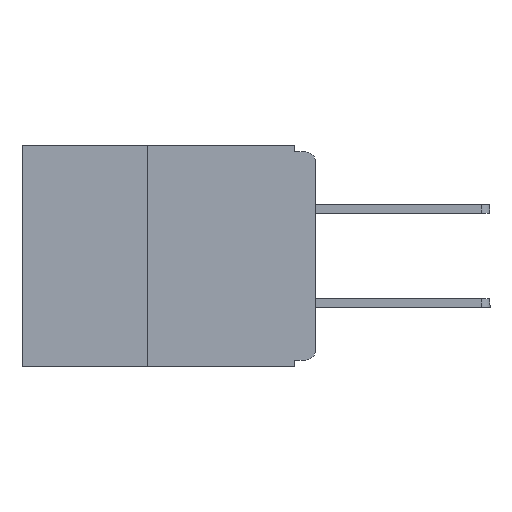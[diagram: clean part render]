
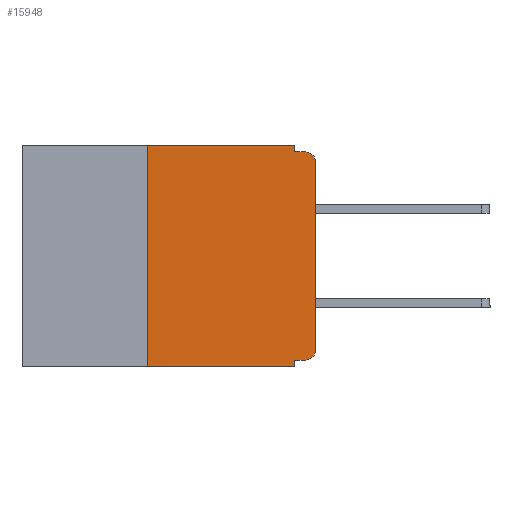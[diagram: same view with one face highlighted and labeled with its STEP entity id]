
A CAD part, left-side view. The second image highlights one B-rep face of the part: STEP entity #15948.
In plain terms, the highlighted planar face has unit normal (-1, 0, 0).
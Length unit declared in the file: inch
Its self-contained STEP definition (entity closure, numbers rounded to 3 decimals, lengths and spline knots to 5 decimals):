
#12 = ORIENTED_EDGE ( 'NONE', *, *, #6398, .T. ) ;
#51 = AXIS2_PLACEMENT_3D ( 'NONE', #2650, #11735, #3995 ) ;
#487 = LINE ( 'NONE', #12885, #13977 ) ;
#543 = CARTESIAN_POINT ( 'NONE',  ( 0., 0.031, -0.32 ) ) ;
#725 = EDGE_CURVE ( 'NONE', #6423, #3817, #10867, .T. ) ;
#857 = CARTESIAN_POINT ( 'NONE',  ( 0., 0.031, -0.33 ) ) ;
#880 = CARTESIAN_POINT ( 'NONE',  ( 0., 0., -0.01 ) ) ;
#1015 = VERTEX_POINT ( 'NONE', #11049 ) ;
#1126 = EDGE_CURVE ( 'NONE', #16452, #16335, #16360, .T. ) ;
#1258 = VERTEX_POINT ( 'NONE', #5091 ) ;
#1505 = VECTOR ( 'NONE', #9692, 39.37008 ) ;
#2023 = VERTEX_POINT ( 'NONE', #8123 ) ;
#2513 = DIRECTION ( 'NONE',  ( 0., 0., 1. ) ) ;
#2650 = CARTESIAN_POINT ( 'NONE',  ( 0., 0.015, -0.025 ) ) ;
#2837 = ORIENTED_EDGE ( 'NONE', *, *, #14425, .T. ) ;
#2912 = CARTESIAN_POINT ( 'NONE',  ( 0., 0.437, -0.33 ) ) ;
#3215 = DIRECTION ( 'NONE',  ( 0., 0., -1. ) ) ;
#3706 = EDGE_CURVE ( 'NONE', #16335, #1015, #5524, .T. ) ;
#3817 = VERTEX_POINT ( 'NONE', #857 ) ;
#3995 = DIRECTION ( 'NONE',  ( 0., 0., -1. ) ) ;
#4114 = CARTESIAN_POINT ( 'NONE',  ( 0., 0., 0. ) ) ;
#4115 = VERTEX_POINT ( 'NONE', #8576 ) ;
#4222 = VECTOR ( 'NONE', #12394, 39.37008 ) ;
#4335 = ORIENTED_EDGE ( 'NONE', *, *, #16655, .T. ) ;
#4448 = ORIENTED_EDGE ( 'NONE', *, *, #15796, .F. ) ;
#4653 = FACE_OUTER_BOUND ( 'NONE', #13528, .T. ) ;
#4668 = EDGE_CURVE ( 'NONE', #1015, #14729, #10681, .T. ) ;
#4706 = DIRECTION ( 'NONE',  ( 0., 0., 1. ) ) ;
#4980 = VECTOR ( 'NONE', #2513, 39.37008 ) ;
#5091 = CARTESIAN_POINT ( 'NONE',  ( 0., 0., -0.025 ) ) ;
#5524 = LINE ( 'NONE', #9822, #1505 ) ;
#6228 = DIRECTION ( 'NONE',  ( -1., 0., 0. ) ) ;
#6257 = CARTESIAN_POINT ( 'NONE',  ( 0., 0.437, 0. ) ) ;
#6385 = CARTESIAN_POINT ( 'NONE',  ( 0., 0.437, 0. ) ) ;
#6398 = EDGE_CURVE ( 'NONE', #4115, #1258, #11850, .T. ) ;
#6423 = VERTEX_POINT ( 'NONE', #543 ) ;
#6607 = ORIENTED_EDGE ( 'NONE', *, *, #10593, .F. ) ;
#6704 = DIRECTION ( 'NONE',  ( 0., -1., 0. ) ) ;
#7155 = CARTESIAN_POINT ( 'NONE',  ( 0., 0.031, 0. ) ) ;
#7385 = CARTESIAN_POINT ( 'NONE',  ( 0., 0.25, 0. ) ) ;
#7498 = VECTOR ( 'NONE', #11972, 39.37008 ) ;
#7620 = DIRECTION ( 'NONE',  ( 0., 0., -1. ) ) ;
#8123 = CARTESIAN_POINT ( 'NONE',  ( 0., 0.25, -0.33 ) ) ;
#8529 = ORIENTED_EDGE ( 'NONE', *, *, #15371, .T. ) ;
#8576 = CARTESIAN_POINT ( 'NONE',  ( 0., 0., -0.305 ) ) ;
#8855 = ORIENTED_EDGE ( 'NONE', *, *, #725, .F. ) ;
#9044 = DIRECTION ( 'NONE',  ( 0., 1., 0. ) ) ;
#9251 = VECTOR ( 'NONE', #6704, 39.37008 ) ;
#9282 = ORIENTED_EDGE ( 'NONE', *, *, #4668, .F. ) ;
#9484 = ORIENTED_EDGE ( 'NONE', *, *, #3706, .F. ) ;
#9692 = DIRECTION ( 'NONE',  ( 0., 0., -1. ) ) ;
#9822 = CARTESIAN_POINT ( 'NONE',  ( 0., 0.031, 0. ) ) ;
#9939 = AXIS2_PLACEMENT_3D ( 'NONE', #6385, #15226, #7620 ) ;
#10044 = ORIENTED_EDGE ( 'NONE', *, *, #1126, .F. ) ;
#10365 = VERTEX_POINT ( 'NONE', #16142 ) ;
#10466 = VECTOR ( 'NONE', #3215, 39.37008 ) ;
#10593 = EDGE_CURVE ( 'NONE', #10365, #6423, #487, .T. ) ;
#10681 = LINE ( 'NONE', #880, #4222 ) ;
#10867 = LINE ( 'NONE', #13278, #10466 ) ;
#10918 = VECTOR ( 'NONE', #4706, 39.37008 ) ;
#10933 = LINE ( 'NONE', #2912, #7498 ) ;
#11049 = CARTESIAN_POINT ( 'NONE',  ( 0., 0.031, -0.01 ) ) ;
#11116 = CIRCLE ( 'NONE', #16629, 0.015 ) ;
#11328 = LINE ( 'NONE', #14842, #10918 ) ;
#11735 = DIRECTION ( 'NONE',  ( -1., 0., 0. ) ) ;
#11850 = LINE ( 'NONE', #4114, #4980 ) ;
#11972 = DIRECTION ( 'NONE',  ( 0., -1., 0. ) ) ;
#12394 = DIRECTION ( 'NONE',  ( 0., -1., 0. ) ) ;
#12744 = PLANE ( 'NONE',  #9939 ) ;
#12885 = CARTESIAN_POINT ( 'NONE',  ( 0., 0., -0.32 ) ) ;
#13278 = CARTESIAN_POINT ( 'NONE',  ( 0., 0.031, -0.33 ) ) ;
#13528 = EDGE_LOOP ( 'NONE', ( #12, #4335, #9282, #9484, #10044, #4448, #8529, #8855, #6607, #2837 ) ) ;
#13826 = CARTESIAN_POINT ( 'NONE',  ( 0., 0.015, -0.305 ) ) ;
#13977 = VECTOR ( 'NONE', #9044, 39.37008 ) ;
#14425 = EDGE_CURVE ( 'NONE', #10365, #4115, #11116, .T. ) ;
#14471 = CARTESIAN_POINT ( 'NONE',  ( 0., 0.015, -0.01 ) ) ;
#14729 = VERTEX_POINT ( 'NONE', #14471 ) ;
#14842 = CARTESIAN_POINT ( 'NONE',  ( 0., 0.25, -0.33 ) ) ;
#15080 = DIRECTION ( 'NONE',  ( 0., 0., -1. ) ) ;
#15226 = DIRECTION ( 'NONE',  ( 1., 0., 0. ) ) ;
#15371 = EDGE_CURVE ( 'NONE', #2023, #3817, #10933, .T. ) ;
#15796 = EDGE_CURVE ( 'NONE', #2023, #16452, #11328, .T. ) ;
#15948 = ADVANCED_FACE ( 'NONE', ( #4653 ), #12744, .F. ) ;
#16142 = CARTESIAN_POINT ( 'NONE',  ( 0., 0.015, -0.32 ) ) ;
#16335 = VERTEX_POINT ( 'NONE', #7155 ) ;
#16360 = LINE ( 'NONE', #6257, #9251 ) ;
#16452 = VERTEX_POINT ( 'NONE', #7385 ) ;
#16629 = AXIS2_PLACEMENT_3D ( 'NONE', #13826, #6228, #15080 ) ;
#16655 = EDGE_CURVE ( 'NONE', #1258, #14729, #16724, .T. ) ;
#16724 = CIRCLE ( 'NONE', #51, 0.015 ) ;
